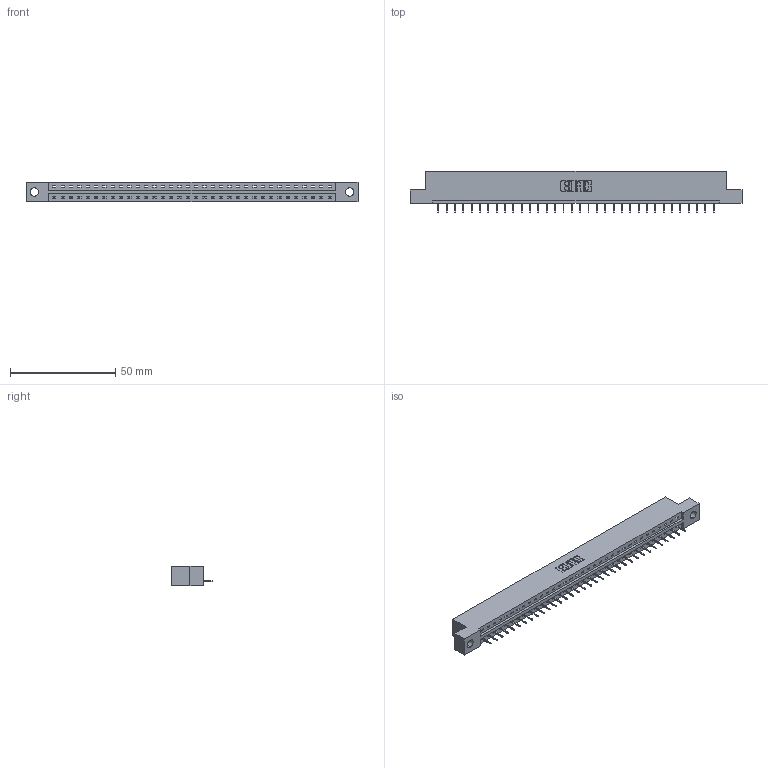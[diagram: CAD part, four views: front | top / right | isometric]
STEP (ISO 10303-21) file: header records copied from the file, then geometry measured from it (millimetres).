
FILE_DESCRIPTION (( 'STEP AP203' ), '1' );
FILE_NAME ('387-034-524-104.STEP', '2018-09-18T12:04:11', ( '' ), ( '' ), 'SwSTEP 2.0', 'SolidWorks 2016', '' );
FILE_SCHEMA (( 'CONFIG_CONTROL_DESIGN' ));
Length unit declared in the file: inch
Products named in the file (3): 345-292-001_345-293-124; 387-034-524-104; 337 Part_Flush Mounting Lugs - 0.156 Dia-TH
Assembly tree (35 placements, depth 2):
  387-034-524-104
    337 Part_Flush Mounting Lugs - 0.156 Dia-TH
    345-292-001_345-293-124  x34
Bounding box: 157.73 x 19.69 x 9.4 mm (x, y, z)
Volume: 16071.5 mm3; surface area: 15886.1 mm2
Topology: 35 solids, 35 shells, 2358 faces, 6839 edges, 4422 vertices
Faces by surface type: plane 1838, cylinder 520
Entity records: 26385 total; most frequent: CARTESIAN_POINT 4600, ORIENTED_EDGE 4570, DIRECTION 3889, EDGE_CURVE 2285, LINE 2161, VECTOR 2161, VERTEX_POINT 1518, AXIS2_PLACEMENT_3D 864
